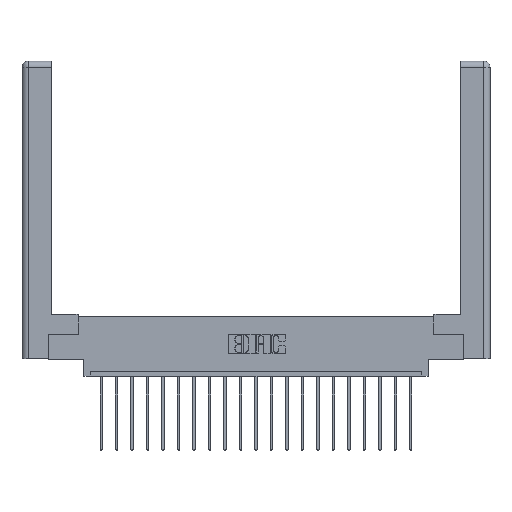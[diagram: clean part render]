
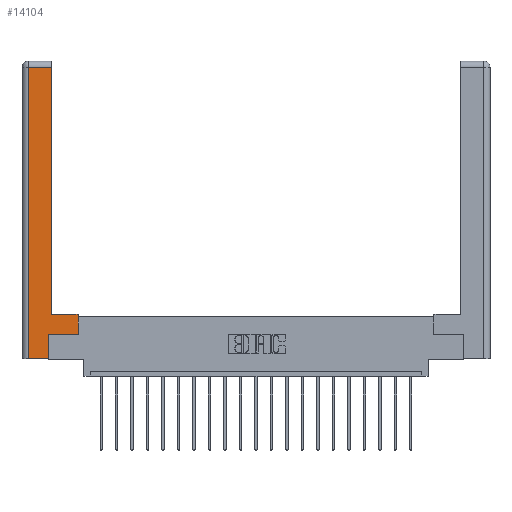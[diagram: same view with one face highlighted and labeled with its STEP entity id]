
A CAD part, top view. The second image highlights one B-rep face of the part: STEP entity #14104.
In plain terms, the highlighted planar face has unit normal (0, 0, 1).
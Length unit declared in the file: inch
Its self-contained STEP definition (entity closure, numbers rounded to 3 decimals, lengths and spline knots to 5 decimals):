
#116 = CARTESIAN_POINT ( 'NONE',  ( 0.565, 0.45, 0. ) ) ;
#816 = ORIENTED_EDGE ( 'NONE', *, *, #17914, .T. ) ;
#859 = VECTOR ( 'NONE', #4066, 39.37008 ) ;
#1075 = EDGE_CURVE ( 'NONE', #18844, #9102, #5024, .T. ) ;
#1260 = EDGE_CURVE ( 'NONE', #1886, #15716, #13604, .T. ) ;
#1390 = VERTEX_POINT ( 'NONE', #17499 ) ;
#1454 = DIRECTION ( 'NONE',  ( -1., 0., 0. ) ) ;
#1540 = EDGE_CURVE ( 'NONE', #1390, #2167, #20532, .T. ) ;
#1876 = CARTESIAN_POINT ( 'NONE',  ( 0.565, 0.245, 0. ) ) ;
#1886 = VERTEX_POINT ( 'NONE', #6541 ) ;
#2167 = VERTEX_POINT ( 'NONE', #17250 ) ;
#2404 = VERTEX_POINT ( 'NONE', #19438 ) ;
#3682 = ORIENTED_EDGE ( 'NONE', *, *, #10145, .T. ) ;
#3983 = PLANE ( 'NONE',  #15976 ) ;
#4066 = DIRECTION ( 'NONE',  ( -1., 0., 0. ) ) ;
#4195 = DIRECTION ( 'NONE',  ( 0., 1., 0. ) ) ;
#4290 = ORIENTED_EDGE ( 'NONE', *, *, #1075, .T. ) ;
#4530 = CARTESIAN_POINT ( 'NONE',  ( 0.265, 0.245, 0. ) ) ;
#4699 = DIRECTION ( 'NONE',  ( 0., -1., 0. ) ) ;
#5016 = LINE ( 'NONE', #13877, #20802 ) ;
#5024 = LINE ( 'NONE', #10548, #21059 ) ;
#5132 = ORIENTED_EDGE ( 'NONE', *, *, #1260, .T. ) ;
#5200 = LINE ( 'NONE', #11925, #859 ) ;
#5621 = VECTOR ( 'NONE', #18017, 39.37008 ) ;
#5652 = DIRECTION ( 'NONE',  ( 0., 1., 0. ) ) ;
#5778 = VECTOR ( 'NONE', #6778, 39.37008 ) ;
#6027 = LINE ( 'NONE', #1876, #5778 ) ;
#6541 = CARTESIAN_POINT ( 'NONE',  ( 0.265, 0., 0. ) ) ;
#6612 = CARTESIAN_POINT ( 'NONE',  ( 0.265, 0., 0. ) ) ;
#6666 = EDGE_CURVE ( 'NONE', #2404, #1886, #14471, .T. ) ;
#6767 = DIRECTION ( 'NONE',  ( 0., 1., 0. ) ) ;
#6778 = DIRECTION ( 'NONE',  ( 1., 0., 0. ) ) ;
#7146 = ORIENTED_EDGE ( 'NONE', *, *, #1540, .T. ) ;
#7219 = DIRECTION ( 'NONE',  ( 0., 0., -1. ) ) ;
#7495 = CARTESIAN_POINT ( 'NONE',  ( 0.295, 0.45, 0. ) ) ;
#8685 = VERTEX_POINT ( 'NONE', #7495 ) ;
#8740 = VECTOR ( 'NONE', #1454, 39.37008 ) ;
#9102 = VERTEX_POINT ( 'NONE', #116 ) ;
#9275 = VECTOR ( 'NONE', #6767, 39.37008 ) ;
#9325 = ORIENTED_EDGE ( 'NONE', *, *, #16000, .T. ) ;
#9642 = CARTESIAN_POINT ( 'NONE',  ( 0.0615, 0., 0. ) ) ;
#10145 = EDGE_CURVE ( 'NONE', #15716, #18844, #6027, .T. ) ;
#10548 = CARTESIAN_POINT ( 'NONE',  ( 0.565, 0.45, 0. ) ) ;
#11159 = EDGE_CURVE ( 'NONE', #8685, #1390, #5016, .T. ) ;
#11621 = ORIENTED_EDGE ( 'NONE', *, *, #11159, .T. ) ;
#11925 = CARTESIAN_POINT ( 'NONE',  ( 0.295, 0.45, 0. ) ) ;
#11970 = FACE_OUTER_BOUND ( 'NONE', #20456, .T. ) ;
#12676 = CARTESIAN_POINT ( 'NONE',  ( 0.0615, 2.94, 0. ) ) ;
#13078 = ORIENTED_EDGE ( 'NONE', *, *, #6666, .T. ) ;
#13417 = CARTESIAN_POINT ( 'NONE',  ( 0.265, 0.245, 0. ) ) ;
#13604 = LINE ( 'NONE', #13417, #9275 ) ;
#13877 = CARTESIAN_POINT ( 'NONE',  ( 0.295, 3., 0. ) ) ;
#13971 = VECTOR ( 'NONE', #4699, 39.37008 ) ;
#14104 = ADVANCED_FACE ( 'NONE', ( #11970 ), #3983, .F. ) ;
#14471 = LINE ( 'NONE', #6612, #5621 ) ;
#14701 = CARTESIAN_POINT ( 'NONE',  ( 0.565, 0.245, 0. ) ) ;
#15308 = CARTESIAN_POINT ( 'NONE',  ( 0., 0., 0. ) ) ;
#15716 = VERTEX_POINT ( 'NONE', #4530 ) ;
#15976 = AXIS2_PLACEMENT_3D ( 'NONE', #15308, #7219, #16830 ) ;
#16000 = EDGE_CURVE ( 'NONE', #9102, #8685, #5200, .T. ) ;
#16830 = DIRECTION ( 'NONE',  ( -1., 0., 0. ) ) ;
#17250 = CARTESIAN_POINT ( 'NONE',  ( 0.0615, 2.94, 0. ) ) ;
#17499 = CARTESIAN_POINT ( 'NONE',  ( 0.295, 2.94, 0. ) ) ;
#17914 = EDGE_CURVE ( 'NONE', #2167, #2404, #19113, .T. ) ;
#18017 = DIRECTION ( 'NONE',  ( 1., 0., 0. ) ) ;
#18844 = VERTEX_POINT ( 'NONE', #14701 ) ;
#19113 = LINE ( 'NONE', #9642, #13971 ) ;
#19438 = CARTESIAN_POINT ( 'NONE',  ( 0.0615, 0., 0. ) ) ;
#20456 = EDGE_LOOP ( 'NONE', ( #11621, #7146, #816, #13078, #5132, #3682, #4290, #9325 ) ) ;
#20532 = LINE ( 'NONE', #12676, #8740 ) ;
#20802 = VECTOR ( 'NONE', #4195, 39.37008 ) ;
#21059 = VECTOR ( 'NONE', #5652, 39.37008 ) ;
